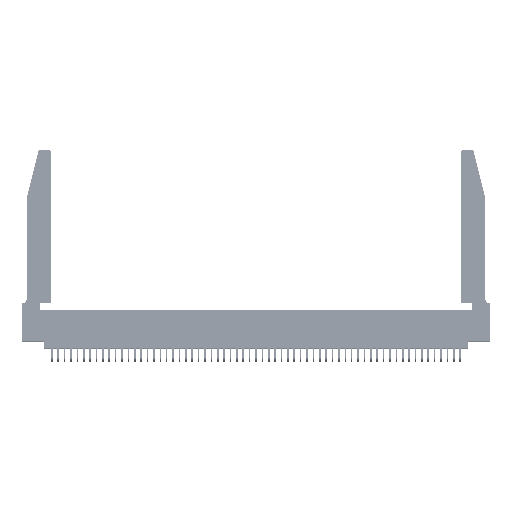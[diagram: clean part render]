
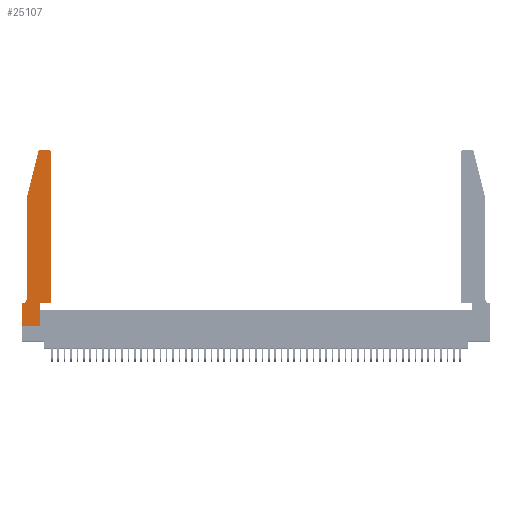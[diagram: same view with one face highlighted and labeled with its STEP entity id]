
A CAD part, top view. The second image highlights one B-rep face of the part: STEP entity #25107.
In plain terms, the highlighted planar face has unit normal (0, 0, 1).
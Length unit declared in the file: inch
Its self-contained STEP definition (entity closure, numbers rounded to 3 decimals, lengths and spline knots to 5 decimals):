
#1324 = LINE ( 'NONE', #46056, #44862 ) ;
#2183 = CARTESIAN_POINT ( 'NONE',  ( 0.2865, 0.35, 0.37 ) ) ;
#2834 = CARTESIAN_POINT ( 'NONE',  ( 0.2865, 0.35, 0.37 ) ) ;
#3321 = CARTESIAN_POINT ( 'NONE',  ( 0.0755, 2., 0.37 ) ) ;
#3649 = VERTEX_POINT ( 'NONE', #19558 ) ;
#4971 = DIRECTION ( 'NONE',  ( 0., 0., 1. ) ) ;
#4974 = CARTESIAN_POINT ( 'NONE',  ( 0.0755, 0.42, 0.37 ) ) ;
#7596 = DIRECTION ( 'NONE',  ( 0., -1., 0. ) ) ;
#8038 = CARTESIAN_POINT ( 'NONE',  ( 0.0755, 2., 0.37 ) ) ;
#8366 = CIRCLE ( 'NONE', #26136, 0.03 ) ;
#8417 = CARTESIAN_POINT ( 'NONE',  ( 0.4505, 0.35, 0.37 ) ) ;
#9716 = EDGE_CURVE ( 'NONE', #12685, #44890, #14916, .T. ) ;
#10446 = EDGE_CURVE ( 'NONE', #27622, #10730, #45054, .T. ) ;
#10620 = EDGE_CURVE ( 'NONE', #16873, #16290, #52180, .T. ) ;
#10730 = VERTEX_POINT ( 'NONE', #4974 ) ;
#11402 = DIRECTION ( 'NONE',  ( 0., 0., -1. ) ) ;
#11476 = VERTEX_POINT ( 'NONE', #39771 ) ;
#11633 = EDGE_CURVE ( 'NONE', #10730, #16873, #52709, .T. ) ;
#12097 = CARTESIAN_POINT ( 'NONE',  ( 0., 0., 0.37 ) ) ;
#12632 = ORIENTED_EDGE ( 'NONE', *, *, #29701, .T. ) ;
#12685 = VERTEX_POINT ( 'NONE', #49827 ) ;
#13173 = VECTOR ( 'NONE', #37566, 39.37008 ) ;
#14630 = VECTOR ( 'NONE', #19253, 39.37008 ) ;
#14916 = LINE ( 'NONE', #2834, #16231 ) ;
#15008 = CARTESIAN_POINT ( 'NONE',  ( 0., 0., 0.37 ) ) ;
#15637 = AXIS2_PLACEMENT_3D ( 'NONE', #27070, #49355, #24270 ) ;
#16231 = VECTOR ( 'NONE', #36674, 39.37008 ) ;
#16290 = VERTEX_POINT ( 'NONE', #38307 ) ;
#16403 = CARTESIAN_POINT ( 'NONE',  ( 0., 0., 0.37 ) ) ;
#16446 = ORIENTED_EDGE ( 'NONE', *, *, #34324, .T. ) ;
#16873 = VERTEX_POINT ( 'NONE', #50605 ) ;
#18678 = CARTESIAN_POINT ( 'NONE',  ( 0.4205, 2.72, 0.37 ) ) ;
#19253 = DIRECTION ( 'NONE',  ( 0., -1., 0. ) ) ;
#19480 = ORIENTED_EDGE ( 'NONE', *, *, #40855, .T. ) ;
#19558 = CARTESIAN_POINT ( 'NONE',  ( 0.4205, 2.75, 0.37 ) ) ;
#19869 = EDGE_CURVE ( 'NONE', #44890, #27701, #1324, .T. ) ;
#22335 = VERTEX_POINT ( 'NONE', #43504 ) ;
#22442 = EDGE_CURVE ( 'NONE', #16290, #47870, #37036, .T. ) ;
#22798 = CARTESIAN_POINT ( 'NONE',  ( 0.4505, 2.72, 0.37 ) ) ;
#22905 = DIRECTION ( 'NONE',  ( 1., 0., 0. ) ) ;
#23265 = ORIENTED_EDGE ( 'NONE', *, *, #45566, .T. ) ;
#24270 = DIRECTION ( 'NONE',  ( 1., 0., 0. ) ) ;
#24378 = ORIENTED_EDGE ( 'NONE', *, *, #22442, .T. ) ;
#24426 = VECTOR ( 'NONE', #42141, 39.37008 ) ;
#25107 = ADVANCED_FACE ( 'NONE', ( #41357 ), #45172, .T. ) ;
#25125 = ORIENTED_EDGE ( 'NONE', *, *, #37177, .T. ) ;
#25307 = LINE ( 'NONE', #44228, #46265 ) ;
#26136 = AXIS2_PLACEMENT_3D ( 'NONE', #18678, #47993, #22905 ) ;
#26855 = LINE ( 'NONE', #12097, #47778 ) ;
#27070 = CARTESIAN_POINT ( 'NONE',  ( 0., 0.35, 0.37 ) ) ;
#27622 = VERTEX_POINT ( 'NONE', #30906 ) ;
#27701 = VERTEX_POINT ( 'NONE', #48008 ) ;
#28110 = CIRCLE ( 'NONE', #33679, 0.03 ) ;
#28545 = ORIENTED_EDGE ( 'NONE', *, *, #19869, .T. ) ;
#29701 = EDGE_CURVE ( 'NONE', #3649, #11476, #25307, .T. ) ;
#30377 = CARTESIAN_POINT ( 'NONE',  ( 0.284, 2.72, 0.37 ) ) ;
#30906 = CARTESIAN_POINT ( 'NONE',  ( 0.0755, 2., 0.37 ) ) ;
#32188 = ORIENTED_EDGE ( 'NONE', *, *, #10620, .T. ) ;
#32679 = VECTOR ( 'NONE', #7596, 39.37008 ) ;
#32890 = ORIENTED_EDGE ( 'NONE', *, *, #10446, .T. ) ;
#33182 = DIRECTION ( 'NONE',  ( 1., 0., 0. ) ) ;
#33448 = AXIS2_PLACEMENT_3D ( 'NONE', #36683, #11402, #40842 ) ;
#33679 = AXIS2_PLACEMENT_3D ( 'NONE', #30377, #4971, #34589 ) ;
#33882 = CARTESIAN_POINT ( 'NONE',  ( 0.0755, 0.35, 0.37 ) ) ;
#34225 = ORIENTED_EDGE ( 'NONE', *, *, #11633, .T. ) ;
#34324 = EDGE_CURVE ( 'NONE', #47870, #12685, #26855, .T. ) ;
#34378 = LINE ( 'NONE', #8417, #24426 ) ;
#34589 = DIRECTION ( 'NONE',  ( 1., 0., 0. ) ) ;
#34996 = ORIENTED_EDGE ( 'NONE', *, *, #43829, .T. ) ;
#35159 = ORIENTED_EDGE ( 'NONE', *, *, #9716, .T. ) ;
#35638 = LINE ( 'NONE', #8038, #13173 ) ;
#36674 = DIRECTION ( 'NONE',  ( 0., 1., 0. ) ) ;
#36683 = CARTESIAN_POINT ( 'NONE',  ( 0.0055, 0.42, 0.37 ) ) ;
#37036 = LINE ( 'NONE', #15008, #14630 ) ;
#37177 = EDGE_CURVE ( 'NONE', #11476, #22335, #28110, .T. ) ;
#37566 = DIRECTION ( 'NONE',  ( -0.239, -0.971, 0. ) ) ;
#38307 = CARTESIAN_POINT ( 'NONE',  ( 0., 0.35, 0.37 ) ) ;
#39771 = CARTESIAN_POINT ( 'NONE',  ( 0.284, 2.75, 0.37 ) ) ;
#40842 = DIRECTION ( 'NONE',  ( -1., 0., 0. ) ) ;
#40855 = EDGE_CURVE ( 'NONE', #22335, #27622, #35638, .T. ) ;
#41357 = FACE_OUTER_BOUND ( 'NONE', #53141, .T. ) ;
#42141 = DIRECTION ( 'NONE',  ( 0., 1., 0. ) ) ;
#43504 = CARTESIAN_POINT ( 'NONE',  ( 0.25487, 2.72718, 0.37 ) ) ;
#43829 = EDGE_CURVE ( 'NONE', #27701, #54123, #34378, .T. ) ;
#44228 = CARTESIAN_POINT ( 'NONE',  ( 0.2605, 2.75, 0.37 ) ) ;
#44862 = VECTOR ( 'NONE', #50249, 39.37008 ) ;
#44890 = VERTEX_POINT ( 'NONE', #2183 ) ;
#45054 = LINE ( 'NONE', #3321, #32679 ) ;
#45172 = PLANE ( 'NONE',  #15637 ) ;
#45566 = EDGE_CURVE ( 'NONE', #54123, #3649, #8366, .T. ) ;
#46056 = CARTESIAN_POINT ( 'NONE',  ( 0.4505, 0.35, 0.37 ) ) ;
#46265 = VECTOR ( 'NONE', #52540, 39.37008 ) ;
#46965 = VECTOR ( 'NONE', #50597, 39.37008 ) ;
#47778 = VECTOR ( 'NONE', #33182, 39.37008 ) ;
#47870 = VERTEX_POINT ( 'NONE', #16403 ) ;
#47993 = DIRECTION ( 'NONE',  ( 0., 0., 1. ) ) ;
#48008 = CARTESIAN_POINT ( 'NONE',  ( 0.4505, 0.35, 0.37 ) ) ;
#49355 = DIRECTION ( 'NONE',  ( 0., 0., 1. ) ) ;
#49827 = CARTESIAN_POINT ( 'NONE',  ( 0.2865, 0., 0.37 ) ) ;
#50249 = DIRECTION ( 'NONE',  ( 1., 0., 0. ) ) ;
#50597 = DIRECTION ( 'NONE',  ( -1., 0., 0. ) ) ;
#50605 = CARTESIAN_POINT ( 'NONE',  ( 0.0055, 0.35, 0.37 ) ) ;
#52180 = LINE ( 'NONE', #33882, #46965 ) ;
#52540 = DIRECTION ( 'NONE',  ( -1., 0., 0. ) ) ;
#52709 = CIRCLE ( 'NONE', #33448, 0.07 ) ;
#53141 = EDGE_LOOP ( 'NONE', ( #12632, #25125, #19480, #32890, #34225, #32188, #24378, #16446, #35159, #28545, #34996, #23265 ) ) ;
#54123 = VERTEX_POINT ( 'NONE', #22798 ) ;
